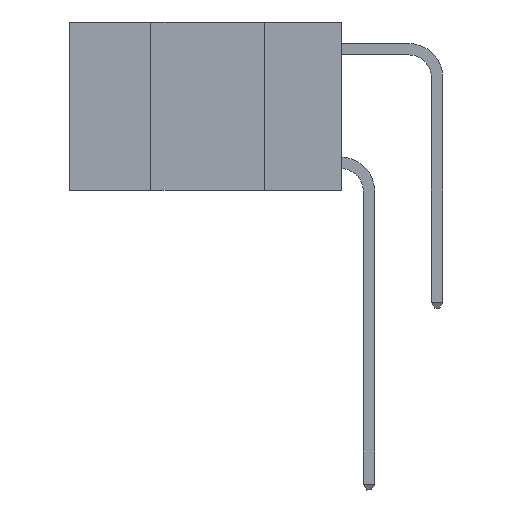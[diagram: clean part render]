
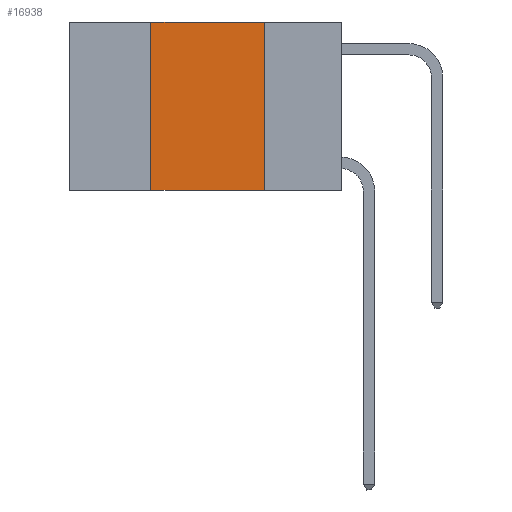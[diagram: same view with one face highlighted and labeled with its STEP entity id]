
A CAD part, left-side view. The second image highlights one B-rep face of the part: STEP entity #16938.
In plain terms, the highlighted planar face has unit normal (-1, 0, 0).
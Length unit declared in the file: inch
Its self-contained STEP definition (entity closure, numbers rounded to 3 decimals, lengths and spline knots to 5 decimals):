
#1425 = DIRECTION ( 'NONE',  ( 0., 0., -1. ) ) ;
#2276 = ORIENTED_EDGE ( 'NONE', *, *, #17321, .T. ) ;
#2369 = CARTESIAN_POINT ( 'NONE',  ( 0., 0.17, 0. ) ) ;
#2665 = ORIENTED_EDGE ( 'NONE', *, *, #3915, .F. ) ;
#2701 = LINE ( 'NONE', #21218, #4705 ) ;
#2856 = CARTESIAN_POINT ( 'NONE',  ( 0., 0.42, 0. ) ) ;
#2898 = VERTEX_POINT ( 'NONE', #19706 ) ;
#3298 = DIRECTION ( 'NONE',  ( 0., 0., 1. ) ) ;
#3755 = LINE ( 'NONE', #10629, #7975 ) ;
#3855 = ORIENTED_EDGE ( 'NONE', *, *, #16018, .F. ) ;
#3915 = EDGE_CURVE ( 'NONE', #10320, #2898, #6329, .T. ) ;
#4705 = VECTOR ( 'NONE', #14655, 39.37008 ) ;
#5028 = ORIENTED_EDGE ( 'NONE', *, *, #12032, .F. ) ;
#5317 = CARTESIAN_POINT ( 'NONE',  ( 0., 0.17, -0.37 ) ) ;
#6238 = DIRECTION ( 'NONE',  ( 1., 0., 0. ) ) ;
#6329 = LINE ( 'NONE', #2856, #16250 ) ;
#7975 = VECTOR ( 'NONE', #10847, 39.37008 ) ;
#10320 = VERTEX_POINT ( 'NONE', #15772 ) ;
#10629 = CARTESIAN_POINT ( 'NONE',  ( 0., 0.6, -0.37 ) ) ;
#10847 = DIRECTION ( 'NONE',  ( 0., -1., 0. ) ) ;
#10859 = AXIS2_PLACEMENT_3D ( 'NONE', #21714, #6238, #1425 ) ;
#12032 = EDGE_CURVE ( 'NONE', #2898, #21336, #16191, .T. ) ;
#13262 = DIRECTION ( 'NONE',  ( 0., -1., 0. ) ) ;
#13645 = EDGE_LOOP ( 'NONE', ( #3855, #5028, #2665, #2276 ) ) ;
#14655 = DIRECTION ( 'NONE',  ( 0., 0., -1. ) ) ;
#15171 = FACE_OUTER_BOUND ( 'NONE', #13645, .T. ) ;
#15772 = CARTESIAN_POINT ( 'NONE',  ( 0., 0.42, -0.37 ) ) ;
#16018 = EDGE_CURVE ( 'NONE', #21336, #17583, #2701, .T. ) ;
#16191 = LINE ( 'NONE', #19581, #18263 ) ;
#16250 = VECTOR ( 'NONE', #3298, 39.37008 ) ;
#16938 = ADVANCED_FACE ( 'NONE', ( #15171 ), #20246, .F. ) ;
#17321 = EDGE_CURVE ( 'NONE', #10320, #17583, #3755, .T. ) ;
#17583 = VERTEX_POINT ( 'NONE', #5317 ) ;
#18263 = VECTOR ( 'NONE', #13262, 39.37008 ) ;
#19581 = CARTESIAN_POINT ( 'NONE',  ( 0., 0.6, 0. ) ) ;
#19706 = CARTESIAN_POINT ( 'NONE',  ( 0., 0.42, 0. ) ) ;
#20246 = PLANE ( 'NONE',  #10859 ) ;
#21218 = CARTESIAN_POINT ( 'NONE',  ( 0., 0.17, 0. ) ) ;
#21336 = VERTEX_POINT ( 'NONE', #2369 ) ;
#21714 = CARTESIAN_POINT ( 'NONE',  ( 0., 0.6, 0. ) ) ;
